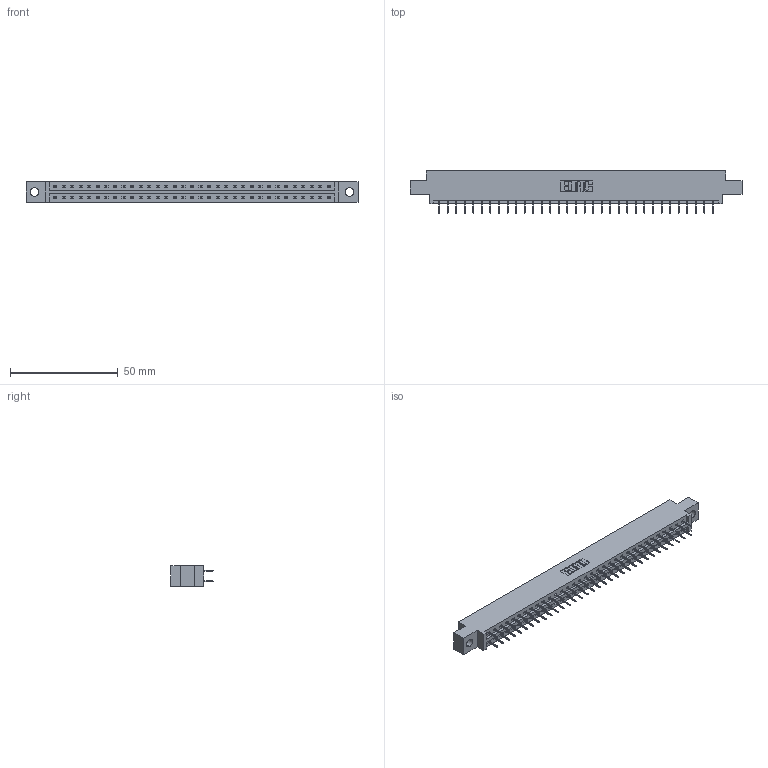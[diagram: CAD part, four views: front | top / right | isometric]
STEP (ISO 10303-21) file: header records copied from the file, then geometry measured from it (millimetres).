
FILE_DESCRIPTION (( 'STEP AP203' ), '1' );
FILE_NAME ('337-066-524-804.STEP', '2019-10-12T00:49:00', ( '' ), ( '' ), 'SwSTEP 2.0', 'SolidWorks 2016', '' );
FILE_SCHEMA (( 'CONFIG_CONTROL_DESIGN' ));
Length unit declared in the file: inch
Products named in the file (3): 345-292-001_345-293-124; 337-066-524-804; 337 Part_0.170 Offset - 0.156 Dia-TH
Assembly tree (67 placements, depth 2):
  337-066-524-804
    337 Part_0.170 Offset - 0.156 Dia-TH
    345-292-001_345-293-124  x66
Bounding box: 153.77 x 19.69 x 9.4 mm (x, y, z)
Volume: 15780.6 mm3; surface area: 17348.5 mm2
Topology: 67 solids, 67 shells, 3946 faces, 11213 edges, 7210 vertices
Faces by surface type: plane 2978, cylinder 968
Entity records: 26959 total; most frequent: CARTESIAN_POINT 4550, ORIENTED_EDGE 4486, DIRECTION 3887, EDGE_CURVE 2243, VECTOR 2119, LINE 2119, VERTEX_POINT 1490, AXIS2_PLACEMENT_3D 884
